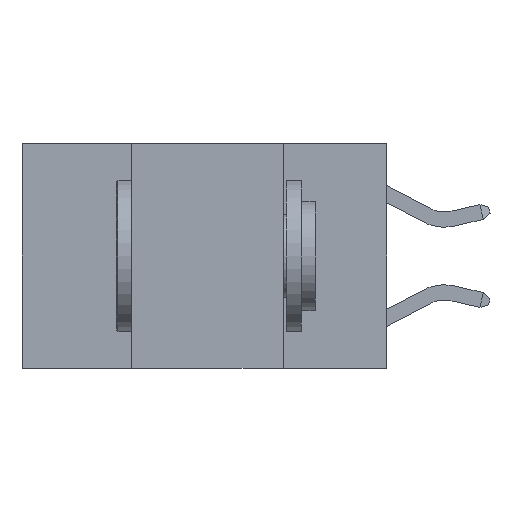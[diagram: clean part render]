
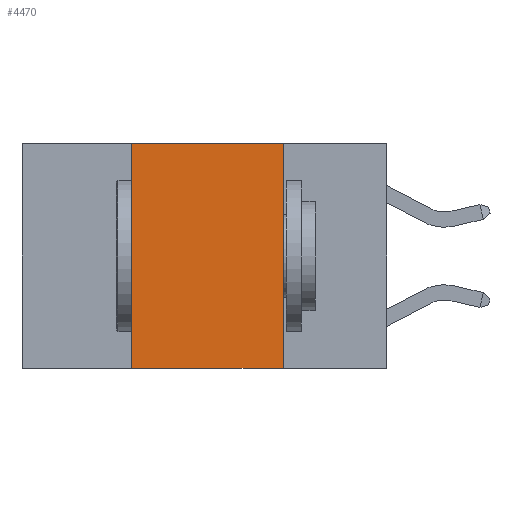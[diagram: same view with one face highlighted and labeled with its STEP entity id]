
A CAD part, left-side view. The second image highlights one B-rep face of the part: STEP entity #4470.
In plain terms, the highlighted planar face has unit normal (-1, 0, 0).
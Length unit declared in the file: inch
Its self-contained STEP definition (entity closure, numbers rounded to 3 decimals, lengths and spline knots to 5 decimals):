
#769 = VERTEX_POINT ( 'NONE', #9034 ) ;
#897 = EDGE_CURVE ( 'NONE', #3320, #3193, #10507, .T. ) ;
#1060 = CARTESIAN_POINT ( 'NONE',  ( 0., 0.6, 0. ) ) ;
#1635 = CARTESIAN_POINT ( 'NONE',  ( 0., 0.42, -0.37 ) ) ;
#2042 = DIRECTION ( 'NONE',  ( 0., -1., 0. ) ) ;
#2781 = CARTESIAN_POINT ( 'NONE',  ( 0., 0.17, 0. ) ) ;
#3102 = ORIENTED_EDGE ( 'NONE', *, *, #897, .F. ) ;
#3193 = VERTEX_POINT ( 'NONE', #13280 ) ;
#3320 = VERTEX_POINT ( 'NONE', #11107 ) ;
#3775 = DIRECTION ( 'NONE',  ( 0., 0., -1. ) ) ;
#4269 = DIRECTION ( 'NONE',  ( 0., -1., 0. ) ) ;
#4470 = ADVANCED_FACE ( 'NONE', ( #4510 ), #8328, .F. ) ;
#4510 = FACE_OUTER_BOUND ( 'NONE', #12656, .T. ) ;
#5045 = LINE ( 'NONE', #5204, #7697 ) ;
#5204 = CARTESIAN_POINT ( 'NONE',  ( 0., 0.42, 0. ) ) ;
#7697 = VECTOR ( 'NONE', #14336, 39.37008 ) ;
#7813 = CARTESIAN_POINT ( 'NONE',  ( 0., 0.6, -0.37 ) ) ;
#7969 = VERTEX_POINT ( 'NONE', #1635 ) ;
#8015 = LINE ( 'NONE', #7813, #8375 ) ;
#8328 = PLANE ( 'NONE',  #8748 ) ;
#8375 = VECTOR ( 'NONE', #2042, 39.37008 ) ;
#8748 = AXIS2_PLACEMENT_3D ( 'NONE', #9457, #10640, #3775 ) ;
#9034 = CARTESIAN_POINT ( 'NONE',  ( 0., 0.17, -0.37 ) ) ;
#9198 = ORIENTED_EDGE ( 'NONE', *, *, #12139, .F. ) ;
#9457 = CARTESIAN_POINT ( 'NONE',  ( 0., 0.6, 0. ) ) ;
#10254 = VECTOR ( 'NONE', #12007, 39.37008 ) ;
#10507 = LINE ( 'NONE', #1060, #13548 ) ;
#10612 = LINE ( 'NONE', #2781, #10254 ) ;
#10640 = DIRECTION ( 'NONE',  ( 1., 0., 0. ) ) ;
#11107 = CARTESIAN_POINT ( 'NONE',  ( 0., 0.42, 0. ) ) ;
#11366 = EDGE_CURVE ( 'NONE', #3193, #769, #10612, .T. ) ;
#12007 = DIRECTION ( 'NONE',  ( 0., 0., -1. ) ) ;
#12139 = EDGE_CURVE ( 'NONE', #7969, #3320, #5045, .T. ) ;
#12656 = EDGE_LOOP ( 'NONE', ( #14577, #3102, #9198, #12985 ) ) ;
#12985 = ORIENTED_EDGE ( 'NONE', *, *, #14343, .T. ) ;
#13280 = CARTESIAN_POINT ( 'NONE',  ( 0., 0.17, 0. ) ) ;
#13548 = VECTOR ( 'NONE', #4269, 39.37008 ) ;
#14336 = DIRECTION ( 'NONE',  ( 0., 0., 1. ) ) ;
#14343 = EDGE_CURVE ( 'NONE', #7969, #769, #8015, .T. ) ;
#14577 = ORIENTED_EDGE ( 'NONE', *, *, #11366, .F. ) ;
